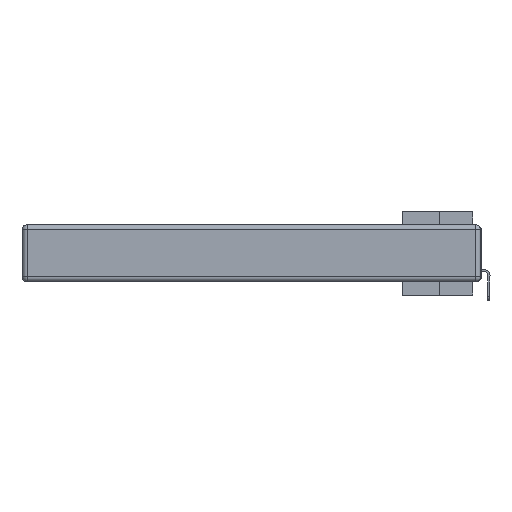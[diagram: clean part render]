
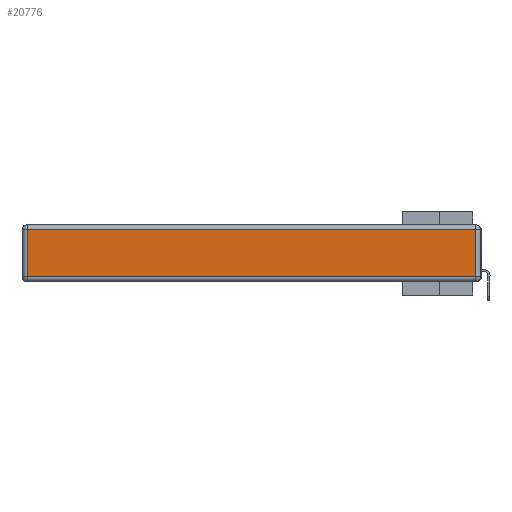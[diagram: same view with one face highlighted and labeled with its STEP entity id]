
A CAD part, left-side view. The second image highlights one B-rep face of the part: STEP entity #20776.
In plain terms, the highlighted planar face has unit normal (-1, 0, 0).
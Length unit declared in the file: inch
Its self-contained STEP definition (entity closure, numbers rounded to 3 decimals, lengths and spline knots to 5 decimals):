
#327 = VERTEX_POINT ( 'NONE', #25931 ) ;
#2081 = DIRECTION ( 'NONE',  ( 0., -1., 0. ) ) ;
#2679 = VECTOR ( 'NONE', #2081, 39.37008 ) ;
#3276 = VERTEX_POINT ( 'NONE', #5535 ) ;
#5052 = EDGE_LOOP ( 'NONE', ( #26782, #26853, #35697, #32618 ) ) ;
#5535 = CARTESIAN_POINT ( 'NONE',  ( 0., 0.03, -0.313 ) ) ;
#5916 = DIRECTION ( 'NONE',  ( 0., 0., -1. ) ) ;
#6485 = CARTESIAN_POINT ( 'NONE',  ( 0., 0.03, -0.343 ) ) ;
#7737 = LINE ( 'NONE', #20847, #33493 ) ;
#8032 = CARTESIAN_POINT ( 'NONE',  ( 0., 2.75, -0.03 ) ) ;
#9837 = DIRECTION ( 'NONE',  ( 0., 0., 1. ) ) ;
#12219 = LINE ( 'NONE', #6485, #14055 ) ;
#14055 = VECTOR ( 'NONE', #9837, 39.37008 ) ;
#14288 = PLANE ( 'NONE',  #23639 ) ;
#14541 = CARTESIAN_POINT ( 'NONE',  ( 0., 0., -0.343 ) ) ;
#17680 = EDGE_CURVE ( 'NONE', #18916, #29663, #35232, .T. ) ;
#18916 = VERTEX_POINT ( 'NONE', #34444 ) ;
#19562 = VECTOR ( 'NONE', #22310, 39.37008 ) ;
#20776 = ADVANCED_FACE ( 'NONE', ( #21992 ), #14288, .T. ) ;
#20847 = CARTESIAN_POINT ( 'NONE',  ( 0., 2.72, -0.343 ) ) ;
#20916 = EDGE_CURVE ( 'NONE', #29663, #327, #7737, .T. ) ;
#21992 = FACE_OUTER_BOUND ( 'NONE', #5052, .T. ) ;
#22310 = DIRECTION ( 'NONE',  ( 0., 1., 0. ) ) ;
#23639 = AXIS2_PLACEMENT_3D ( 'NONE', #14541, #34639, #28741 ) ;
#24340 = LINE ( 'NONE', #37363, #2679 ) ;
#25681 = CARTESIAN_POINT ( 'NONE',  ( 0., 2.72, -0.03 ) ) ;
#25931 = CARTESIAN_POINT ( 'NONE',  ( 0., 2.72, -0.313 ) ) ;
#26782 = ORIENTED_EDGE ( 'NONE', *, *, #32958, .T. ) ;
#26853 = ORIENTED_EDGE ( 'NONE', *, *, #34557, .T. ) ;
#28741 = DIRECTION ( 'NONE',  ( 0., 0., 1. ) ) ;
#29663 = VERTEX_POINT ( 'NONE', #25681 ) ;
#32618 = ORIENTED_EDGE ( 'NONE', *, *, #20916, .T. ) ;
#32958 = EDGE_CURVE ( 'NONE', #327, #3276, #24340, .T. ) ;
#33493 = VECTOR ( 'NONE', #5916, 39.37008 ) ;
#34444 = CARTESIAN_POINT ( 'NONE',  ( 0., 0.03, -0.03 ) ) ;
#34557 = EDGE_CURVE ( 'NONE', #3276, #18916, #12219, .T. ) ;
#34639 = DIRECTION ( 'NONE',  ( -1., 0., 0. ) ) ;
#35232 = LINE ( 'NONE', #8032, #19562 ) ;
#35697 = ORIENTED_EDGE ( 'NONE', *, *, #17680, .T. ) ;
#37363 = CARTESIAN_POINT ( 'NONE',  ( 0., 0., -0.313 ) ) ;
